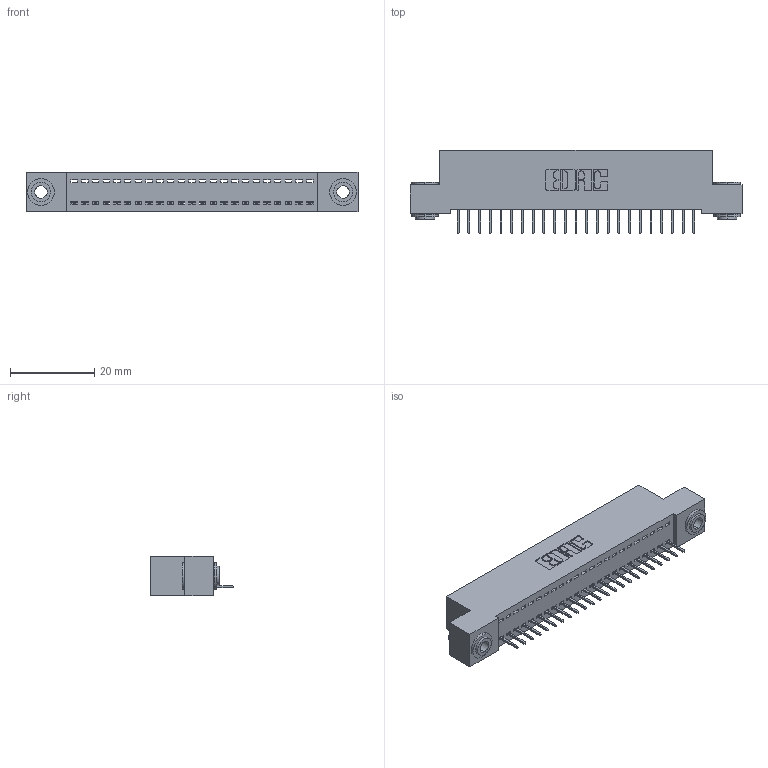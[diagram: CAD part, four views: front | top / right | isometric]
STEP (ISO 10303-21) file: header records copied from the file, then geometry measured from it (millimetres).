
FILE_DESCRIPTION (( 'STEP AP203' ), '1' );
FILE_NAME ('392-023-524-103.STEP', '2018-08-15T13:24:29', ( '' ), ( '' ), 'SwSTEP 2.0', 'SolidWorks 2016', '' );
FILE_SCHEMA (( 'CONFIG_CONTROL_DESIGN' ));
Length unit declared in the file: inch
Products named in the file (4): 342 Part_.156 TH; 345-292-001_345-293-124; 342-250-002_345-250-002-102; 392-023-524-103
Assembly tree (26 placements, depth 2):
  392-023-524-103
    342 Part_.156 TH
    345-292-001_345-293-124  x23
    342-250-002_345-250-002-102  x2
Bounding box: 78.74 x 19.69 x 9.4 mm (x, y, z)
Volume: 6765.9 mm3; surface area: 9524.6 mm2
Topology: 26 solids, 26 shells, 1574 faces, 4515 edges, 2914 vertices
Faces by surface type: plane 1180, cylinder 386, cone 8
Entity records: 17110 total; most frequent: CARTESIAN_POINT 2930, ORIENTED_EDGE 2882, DIRECTION 2545, EDGE_CURVE 1441, VECTOR 1293, LINE 1293, VERTEX_POINT 954, AXIS2_PLACEMENT_3D 626
